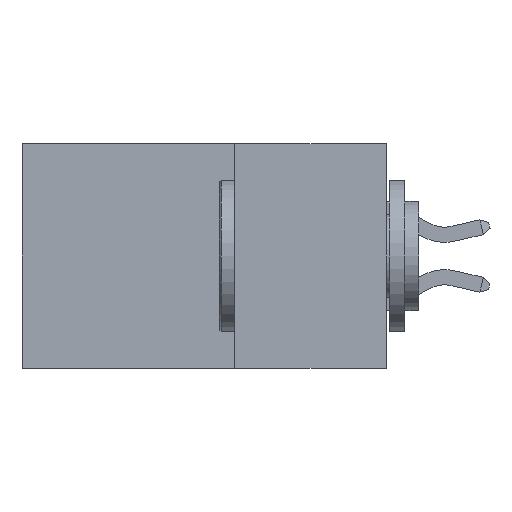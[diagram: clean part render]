
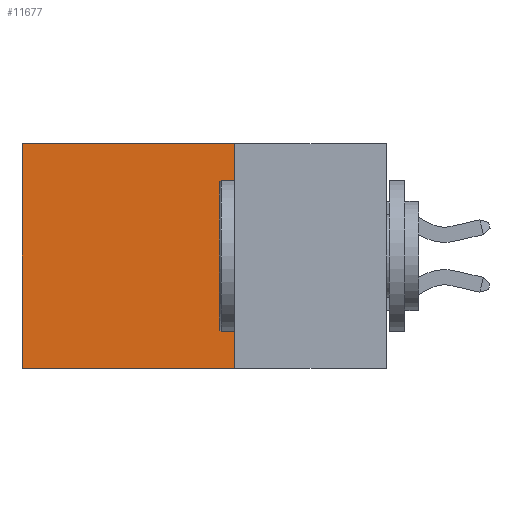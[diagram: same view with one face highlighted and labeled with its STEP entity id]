
A CAD part, left-side view. The second image highlights one B-rep face of the part: STEP entity #11677.
In plain terms, the highlighted planar face has unit normal (-1, 0, 0).
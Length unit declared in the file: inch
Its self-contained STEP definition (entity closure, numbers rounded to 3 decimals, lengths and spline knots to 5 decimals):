
#78 = VECTOR ( 'NONE', #14273, 39.37008 ) ;
#651 = DIRECTION ( 'NONE',  ( 0., 1., 0. ) ) ;
#892 = PLANE ( 'NONE',  #14650 ) ;
#2000 = ORIENTED_EDGE ( 'NONE', *, *, #8850, .F. ) ;
#2263 = VERTEX_POINT ( 'NONE', #28300 ) ;
#3535 = CARTESIAN_POINT ( 'NONE',  ( 0.298, 0.25, 0. ) ) ;
#3829 = LINE ( 'NONE', #6297, #21461 ) ;
#4680 = VERTEX_POINT ( 'NONE', #18272 ) ;
#5778 = VECTOR ( 'NONE', #5851, 39.37008 ) ;
#5851 = DIRECTION ( 'NONE',  ( 0., 1., 0. ) ) ;
#6138 = LINE ( 'NONE', #27837, #78 ) ;
#6297 = CARTESIAN_POINT ( 'NONE',  ( 0.298, 0.25, 0. ) ) ;
#7534 = ORIENTED_EDGE ( 'NONE', *, *, #14249, .F. ) ;
#8603 = DIRECTION ( 'NONE',  ( 0., 0., -1. ) ) ;
#8850 = EDGE_CURVE ( 'NONE', #4680, #22838, #3829, .T. ) ;
#10093 = DIRECTION ( 'NONE',  ( 1., 0., 0. ) ) ;
#11677 = ADVANCED_FACE ( 'NONE', ( #18393 ), #892, .F. ) ;
#12086 = EDGE_CURVE ( 'NONE', #21299, #2263, #6138, .T. ) ;
#12642 = CARTESIAN_POINT ( 'NONE',  ( 0.298, 0.6, 0. ) ) ;
#14249 = EDGE_CURVE ( 'NONE', #22838, #2263, #21830, .T. ) ;
#14273 = DIRECTION ( 'NONE',  ( 0., 0., -1. ) ) ;
#14650 = AXIS2_PLACEMENT_3D ( 'NONE', #23867, #10093, #26108 ) ;
#16702 = CARTESIAN_POINT ( 'NONE',  ( 0.298, 0.25, -0.37 ) ) ;
#17623 = CARTESIAN_POINT ( 'NONE',  ( 0.298, 0.25, -0.37 ) ) ;
#18272 = CARTESIAN_POINT ( 'NONE',  ( 0.298, 0.25, 0. ) ) ;
#18393 = FACE_OUTER_BOUND ( 'NONE', #24991, .T. ) ;
#19353 = ORIENTED_EDGE ( 'NONE', *, *, #12086, .T. ) ;
#20387 = VECTOR ( 'NONE', #651, 39.37008 ) ;
#21299 = VERTEX_POINT ( 'NONE', #12642 ) ;
#21461 = VECTOR ( 'NONE', #8603, 39.37008 ) ;
#21830 = LINE ( 'NONE', #16702, #20387 ) ;
#22730 = EDGE_CURVE ( 'NONE', #4680, #21299, #24130, .T. ) ;
#22838 = VERTEX_POINT ( 'NONE', #17623 ) ;
#23867 = CARTESIAN_POINT ( 'NONE',  ( 0.298, 0.25, 0. ) ) ;
#24130 = LINE ( 'NONE', #3535, #5778 ) ;
#24991 = EDGE_LOOP ( 'NONE', ( #19353, #7534, #2000, #27729 ) ) ;
#26108 = DIRECTION ( 'NONE',  ( 0., 0., -1. ) ) ;
#27729 = ORIENTED_EDGE ( 'NONE', *, *, #22730, .T. ) ;
#27837 = CARTESIAN_POINT ( 'NONE',  ( 0.298, 0.6, 0. ) ) ;
#28300 = CARTESIAN_POINT ( 'NONE',  ( 0.298, 0.6, -0.37 ) ) ;
